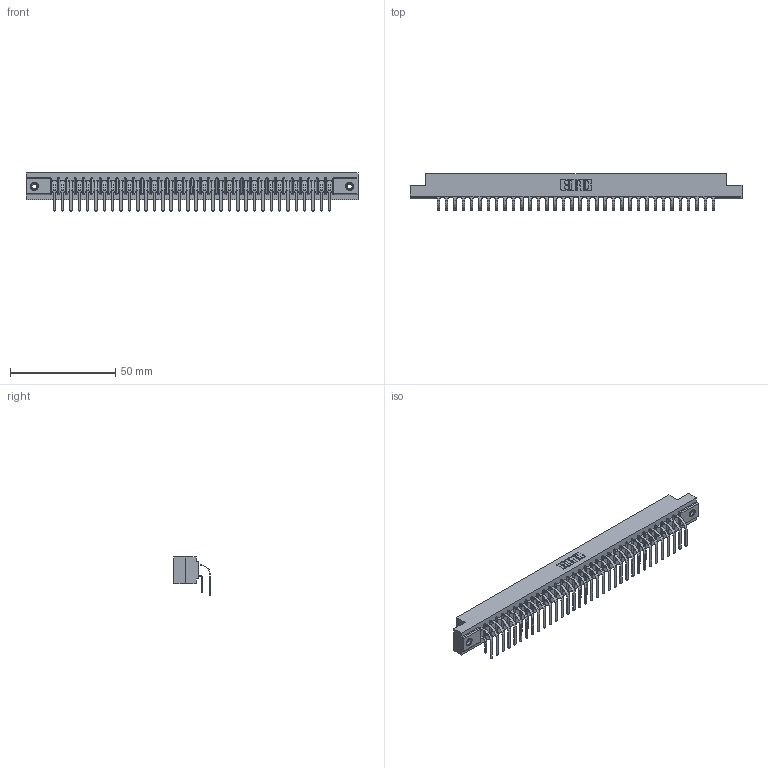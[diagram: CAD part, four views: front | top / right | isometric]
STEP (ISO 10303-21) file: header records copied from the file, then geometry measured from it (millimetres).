
FILE_DESCRIPTION (( 'STEP AP203' ), '1' );
FILE_NAME ('307-068-459-208.STEP', '2022-07-07T18:35:13', ( '' ), ( '' ), 'SwSTEP 2.0', 'SolidWorks 2020', '' );
FILE_SCHEMA (( 'CONFIG_CONTROL_DESIGN' ));
Length unit declared in the file: inch
Products named in the file (5): 307-068-459-208; 345-250-001_345-250-003-102; 307-290-001_559 - 2 (Single); 307 Part_.156 Dia Mounting Holes; 307-290-001_558 559 - 1 (Single)
Assembly tree (71 placements, depth 2):
  307-068-459-208
    307 Part_.156 Dia Mounting Holes
    307-290-001_558 559 - 1 (Single)  x34
    307-290-001_559 - 2 (Single)  x34
    345-250-001_345-250-003-102  x2
Bounding box: 157.73 x 17.51 x 18.07 mm (x, y, z)
Volume: 16965.7 mm3; surface area: 22074.7 mm2
Topology: 71 solids, 71 shells, 3613 faces, 10115 edges, 6550 vertices
Faces by surface type: plane 2346, cylinder 1181, sphere 70, cone 12, torus 4
Entity records: 33854 total; most frequent: CARTESIAN_POINT 5527, ORIENTED_EDGE 5470, DIRECTION 5425, EDGE_CURVE 2735, LINE 2093, VECTOR 2093, VERTEX_POINT 1768, AXIS2_PLACEMENT_3D 1666
